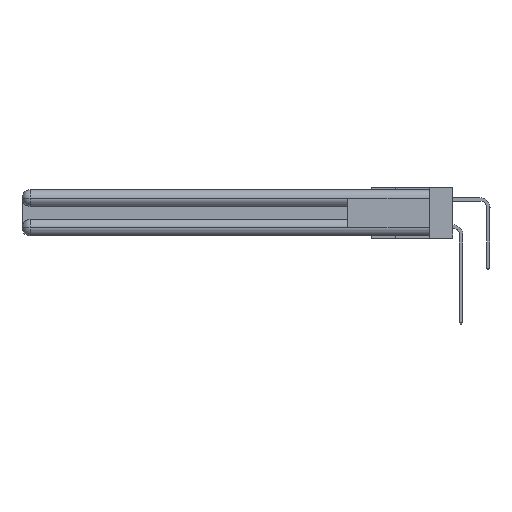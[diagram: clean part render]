
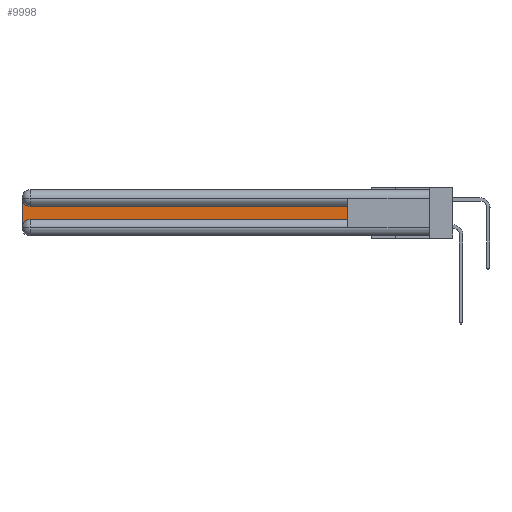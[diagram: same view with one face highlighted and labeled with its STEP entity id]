
A CAD part, left-side view. The second image highlights one B-rep face of the part: STEP entity #9998.
In plain terms, the highlighted planar face has unit normal (-1, 0, 0).
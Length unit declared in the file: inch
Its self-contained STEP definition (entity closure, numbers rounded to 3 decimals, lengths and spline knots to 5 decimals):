
#631 = CARTESIAN_POINT ( 'NONE',  ( 0.075, 0.6, -0.2175 ) ) ;
#2528 = EDGE_CURVE ( 'NONE', #27579, #5702, #10833, .T. ) ;
#2655 = DIRECTION ( 'NONE',  ( 0., 1., 0. ) ) ;
#3111 = VECTOR ( 'NONE', #2655, 39.37008 ) ;
#3246 = LINE ( 'NONE', #631, #10430 ) ;
#4461 = DIRECTION ( 'NONE',  ( 1., 0., 0. ) ) ;
#4589 = CARTESIAN_POINT ( 'NONE',  ( 0.075, 2.94, -0.2775 ) ) ;
#4641 = CARTESIAN_POINT ( 'NONE',  ( 0.075, 3., -0.2775 ) ) ;
#4680 = CARTESIAN_POINT ( 'NONE',  ( 0.075, 3., -0.1225 ) ) ;
#5124 = AXIS2_PLACEMENT_3D ( 'NONE', #4680, #16054, #16315 ) ;
#5343 = CARTESIAN_POINT ( 'NONE',  ( 0.075, 2.94, -0.0625 ) ) ;
#5458 = EDGE_CURVE ( 'NONE', #23747, #6679, #30789, .T. ) ;
#5702 = VERTEX_POINT ( 'NONE', #25433 ) ;
#6441 = DIRECTION ( 'NONE',  ( 0., 0., -1. ) ) ;
#6679 = VERTEX_POINT ( 'NONE', #18682 ) ;
#8574 = AXIS2_PLACEMENT_3D ( 'NONE', #4589, #4461, #36427 ) ;
#9210 = DIRECTION ( 'NONE',  ( 1., 0., 0. ) ) ;
#9469 = ORIENTED_EDGE ( 'NONE', *, *, #34559, .T. ) ;
#9998 = ADVANCED_FACE ( 'NONE', ( #27605 ), #21726, .F. ) ;
#10430 = VECTOR ( 'NONE', #32626, 39.37008 ) ;
#10833 = LINE ( 'NONE', #36620, #22494 ) ;
#11166 = DIRECTION ( 'NONE',  ( 0., 0., 1. ) ) ;
#12014 = ORIENTED_EDGE ( 'NONE', *, *, #20355, .T. ) ;
#12020 = EDGE_CURVE ( 'NONE', #34162, #36666, #28400, .T. ) ;
#13459 = LINE ( 'NONE', #20270, #29635 ) ;
#16054 = DIRECTION ( 'NONE',  ( 1., 0., 0. ) ) ;
#16315 = DIRECTION ( 'NONE',  ( 0., 0., -1. ) ) ;
#16632 = AXIS2_PLACEMENT_3D ( 'NONE', #5343, #9210, #6441 ) ;
#18302 = ORIENTED_EDGE ( 'NONE', *, *, #5458, .T. ) ;
#18682 = CARTESIAN_POINT ( 'NONE',  ( 0.075, 2.94, -0.2175 ) ) ;
#20270 = CARTESIAN_POINT ( 'NONE',  ( 0.075, 3., -0.2175 ) ) ;
#20355 = EDGE_CURVE ( 'NONE', #6679, #27579, #3246, .T. ) ;
#20401 = DIRECTION ( 'NONE',  ( 0., 0., -1. ) ) ;
#21426 = EDGE_LOOP ( 'NONE', ( #9469, #28342, #33327, #18302, #12014, #26971 ) ) ;
#21726 = PLANE ( 'NONE',  #5124 ) ;
#21832 = CARTESIAN_POINT ( 'NONE',  ( 0.075, 3., -0.0625 ) ) ;
#22494 = VECTOR ( 'NONE', #11166, 39.37008 ) ;
#23239 = CARTESIAN_POINT ( 'NONE',  ( 0.075, 0.6, -0.1225 ) ) ;
#23747 = VERTEX_POINT ( 'NONE', #4641 ) ;
#24247 = CARTESIAN_POINT ( 'NONE',  ( 0.075, 2.94, -0.1225 ) ) ;
#24518 = CARTESIAN_POINT ( 'NONE',  ( 0.075, 0.6, -0.2175 ) ) ;
#25433 = CARTESIAN_POINT ( 'NONE',  ( 0.075, 0.6, -0.1225 ) ) ;
#26971 = ORIENTED_EDGE ( 'NONE', *, *, #2528, .T. ) ;
#27579 = VERTEX_POINT ( 'NONE', #24518 ) ;
#27605 = FACE_OUTER_BOUND ( 'NONE', #21426, .T. ) ;
#28342 = ORIENTED_EDGE ( 'NONE', *, *, #12020, .T. ) ;
#28400 = CIRCLE ( 'NONE', #16632, 0.06 ) ;
#28945 = EDGE_CURVE ( 'NONE', #36666, #23747, #13459, .T. ) ;
#29635 = VECTOR ( 'NONE', #20401, 39.37008 ) ;
#30789 = CIRCLE ( 'NONE', #8574, 0.06 ) ;
#32626 = DIRECTION ( 'NONE',  ( 0., -1., 0. ) ) ;
#33327 = ORIENTED_EDGE ( 'NONE', *, *, #28945, .T. ) ;
#34067 = LINE ( 'NONE', #23239, #3111 ) ;
#34162 = VERTEX_POINT ( 'NONE', #24247 ) ;
#34559 = EDGE_CURVE ( 'NONE', #5702, #34162, #34067, .T. ) ;
#36427 = DIRECTION ( 'NONE',  ( 0., 0., -1. ) ) ;
#36620 = CARTESIAN_POINT ( 'NONE',  ( 0.075, 0.6, -0.2175 ) ) ;
#36666 = VERTEX_POINT ( 'NONE', #21832 ) ;
